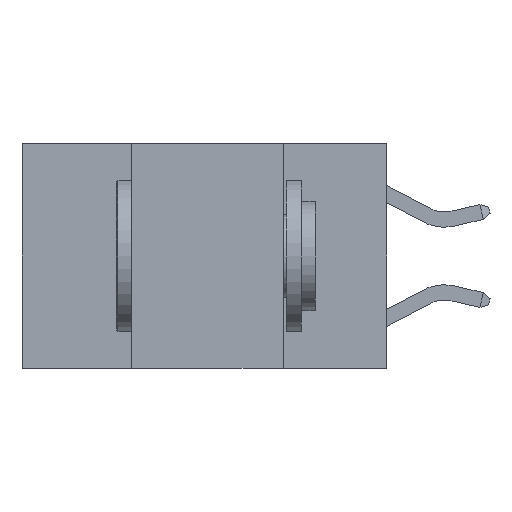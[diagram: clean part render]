
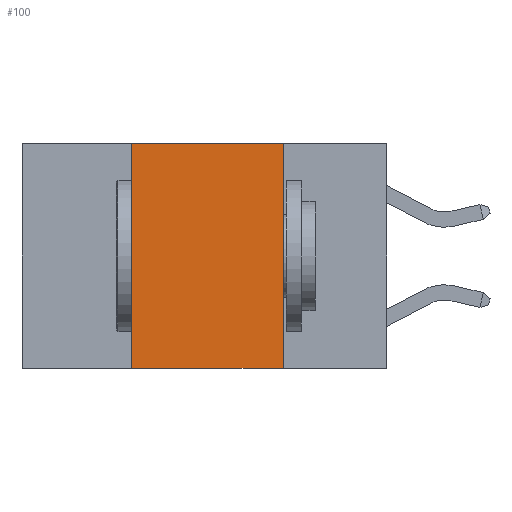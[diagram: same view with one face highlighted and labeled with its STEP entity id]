
A CAD part, left-side view. The second image highlights one B-rep face of the part: STEP entity #100.
In plain terms, the highlighted planar face has unit normal (-1, 0, 0).
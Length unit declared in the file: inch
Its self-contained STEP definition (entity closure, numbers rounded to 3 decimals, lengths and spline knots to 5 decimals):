
#100 = ADVANCED_FACE ( 'NONE', ( #673 ), #7976, .F. ) ;
#367 = EDGE_LOOP ( 'NONE', ( #10875, #21924, #16904, #22842 ) ) ;
#673 = FACE_OUTER_BOUND ( 'NONE', #367, .T. ) ;
#1317 = CARTESIAN_POINT ( 'NONE',  ( 0., 0.42, -0.37 ) ) ;
#1503 = EDGE_CURVE ( 'NONE', #2402, #16106, #15883, .T. ) ;
#2349 = CARTESIAN_POINT ( 'NONE',  ( 0., 0.6, 0. ) ) ;
#2402 = VERTEX_POINT ( 'NONE', #10714 ) ;
#2404 = CARTESIAN_POINT ( 'NONE',  ( 0., 0.17, 0. ) ) ;
#4130 = VECTOR ( 'NONE', #14101, 39.37008 ) ;
#4336 = DIRECTION ( 'NONE',  ( 0., -1., 0. ) ) ;
#5620 = VERTEX_POINT ( 'NONE', #21267 ) ;
#6105 = CARTESIAN_POINT ( 'NONE',  ( 0., 0.42, 0. ) ) ;
#6681 = AXIS2_PLACEMENT_3D ( 'NONE', #2349, #16979, #10006 ) ;
#6769 = CARTESIAN_POINT ( 'NONE',  ( 0., 0.6, 0. ) ) ;
#6940 = VERTEX_POINT ( 'NONE', #1317 ) ;
#7746 = CARTESIAN_POINT ( 'NONE',  ( 0., 0.17, 0. ) ) ;
#7976 = PLANE ( 'NONE',  #6681 ) ;
#10006 = DIRECTION ( 'NONE',  ( 0., 0., -1. ) ) ;
#10714 = CARTESIAN_POINT ( 'NONE',  ( 0., 0.42, 0. ) ) ;
#10875 = ORIENTED_EDGE ( 'NONE', *, *, #11581, .F. ) ;
#11132 = EDGE_CURVE ( 'NONE', #6940, #2402, #17026, .T. ) ;
#11139 = DIRECTION ( 'NONE',  ( 0., 0., 1. ) ) ;
#11581 = EDGE_CURVE ( 'NONE', #16106, #5620, #16641, .T. ) ;
#12003 = VECTOR ( 'NONE', #11139, 39.37008 ) ;
#12685 = EDGE_CURVE ( 'NONE', #6940, #5620, #13466, .T. ) ;
#13466 = LINE ( 'NONE', #20753, #20946 ) ;
#14101 = DIRECTION ( 'NONE',  ( 0., -1., 0. ) ) ;
#15797 = VECTOR ( 'NONE', #18639, 39.37008 ) ;
#15883 = LINE ( 'NONE', #6769, #4130 ) ;
#16106 = VERTEX_POINT ( 'NONE', #2404 ) ;
#16641 = LINE ( 'NONE', #7746, #15797 ) ;
#16904 = ORIENTED_EDGE ( 'NONE', *, *, #11132, .F. ) ;
#16979 = DIRECTION ( 'NONE',  ( 1., 0., 0. ) ) ;
#17026 = LINE ( 'NONE', #6105, #12003 ) ;
#18639 = DIRECTION ( 'NONE',  ( 0., 0., -1. ) ) ;
#20753 = CARTESIAN_POINT ( 'NONE',  ( 0., 0.6, -0.37 ) ) ;
#20946 = VECTOR ( 'NONE', #4336, 39.37008 ) ;
#21267 = CARTESIAN_POINT ( 'NONE',  ( 0., 0.17, -0.37 ) ) ;
#21924 = ORIENTED_EDGE ( 'NONE', *, *, #1503, .F. ) ;
#22842 = ORIENTED_EDGE ( 'NONE', *, *, #12685, .T. ) ;
